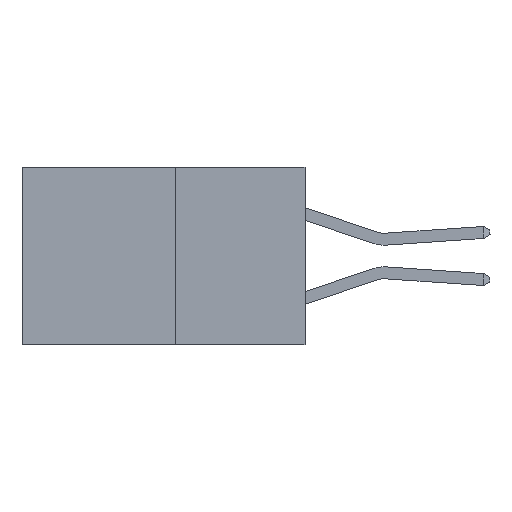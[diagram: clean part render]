
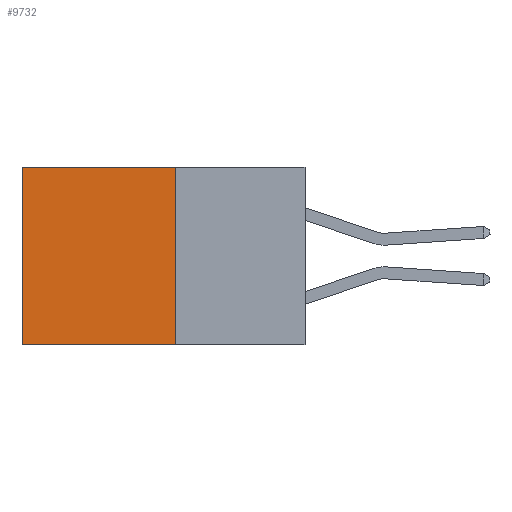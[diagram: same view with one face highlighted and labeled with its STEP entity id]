
A CAD part, left-side view. The second image highlights one B-rep face of the part: STEP entity #9732.
In plain terms, the highlighted planar face has unit normal (-1, 0, 0).
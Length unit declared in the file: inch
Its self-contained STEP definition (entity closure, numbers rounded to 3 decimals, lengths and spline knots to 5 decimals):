
#3064 = VECTOR ( 'NONE', #11258, 39.37008 ) ;
#3318 = LINE ( 'NONE', #26688, #25827 ) ;
#5548 = CARTESIAN_POINT ( 'NONE',  ( 0.277, 0.27, -0.37 ) ) ;
#6165 = EDGE_LOOP ( 'NONE', ( #16351, #18830, #10374, #27273 ) ) ;
#6809 = CARTESIAN_POINT ( 'NONE',  ( 0.277, 0.27, 0. ) ) ;
#8513 = CARTESIAN_POINT ( 'NONE',  ( 0.277, 0.27, 0. ) ) ;
#9732 = ADVANCED_FACE ( 'NONE', ( #14969 ), #10434, .F. ) ;
#10374 = ORIENTED_EDGE ( 'NONE', *, *, #22348, .F. ) ;
#10434 = PLANE ( 'NONE',  #16126 ) ;
#11258 = DIRECTION ( 'NONE',  ( 0., 1., 0. ) ) ;
#11774 = DIRECTION ( 'NONE',  ( 0., 0., -1. ) ) ;
#11923 = VERTEX_POINT ( 'NONE', #13321 ) ;
#12644 = DIRECTION ( 'NONE',  ( 1., 0., 0. ) ) ;
#13321 = CARTESIAN_POINT ( 'NONE',  ( 0.277, 0.59, 0. ) ) ;
#13821 = DIRECTION ( 'NONE',  ( 0., 1., 0. ) ) ;
#14969 = FACE_OUTER_BOUND ( 'NONE', #6165, .T. ) ;
#15957 = DIRECTION ( 'NONE',  ( 0., 0., -1. ) ) ;
#16126 = AXIS2_PLACEMENT_3D ( 'NONE', #25613, #12644, #27761 ) ;
#16318 = VERTEX_POINT ( 'NONE', #22863 ) ;
#16351 = ORIENTED_EDGE ( 'NONE', *, *, #17565, .T. ) ;
#17565 = EDGE_CURVE ( 'NONE', #11923, #16318, #27337, .T. ) ;
#18094 = CARTESIAN_POINT ( 'NONE',  ( 0.277, 0.27, -0.37 ) ) ;
#18254 = CARTESIAN_POINT ( 'NONE',  ( 0.277, 0.59, -0.37 ) ) ;
#18830 = ORIENTED_EDGE ( 'NONE', *, *, #22107, .F. ) ;
#19216 = EDGE_CURVE ( 'NONE', #23349, #11923, #21231, .T. ) ;
#19799 = VECTOR ( 'NONE', #13821, 39.37008 ) ;
#20483 = LINE ( 'NONE', #18094, #19799 ) ;
#21231 = LINE ( 'NONE', #6809, #3064 ) ;
#21518 = VERTEX_POINT ( 'NONE', #5548 ) ;
#21661 = VECTOR ( 'NONE', #11774, 39.37008 ) ;
#22107 = EDGE_CURVE ( 'NONE', #21518, #16318, #20483, .T. ) ;
#22348 = EDGE_CURVE ( 'NONE', #23349, #21518, #3318, .T. ) ;
#22863 = CARTESIAN_POINT ( 'NONE',  ( 0.277, 0.59, -0.37 ) ) ;
#23349 = VERTEX_POINT ( 'NONE', #8513 ) ;
#25613 = CARTESIAN_POINT ( 'NONE',  ( 0.277, 0.27, -0.37 ) ) ;
#25827 = VECTOR ( 'NONE', #15957, 39.37008 ) ;
#26688 = CARTESIAN_POINT ( 'NONE',  ( 0.277, 0.27, -0.37 ) ) ;
#27273 = ORIENTED_EDGE ( 'NONE', *, *, #19216, .T. ) ;
#27337 = LINE ( 'NONE', #18254, #21661 ) ;
#27761 = DIRECTION ( 'NONE',  ( 0., 0., -1. ) ) ;
